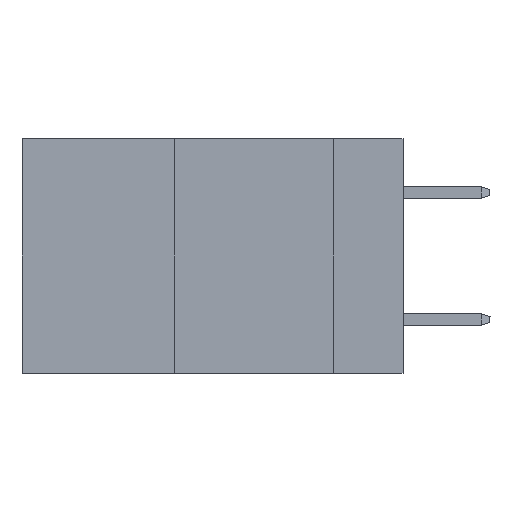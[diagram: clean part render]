
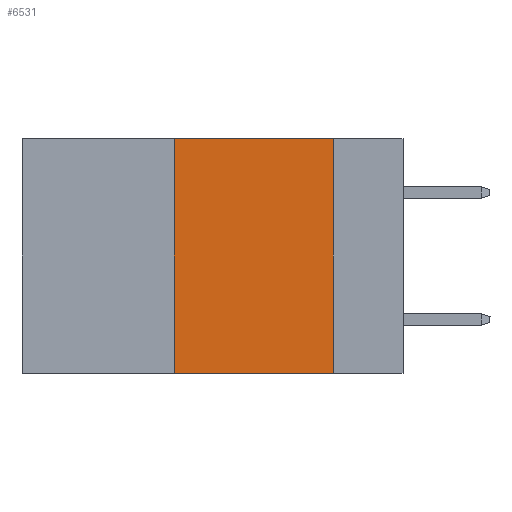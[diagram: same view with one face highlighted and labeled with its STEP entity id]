
A CAD part, left-side view. The second image highlights one B-rep face of the part: STEP entity #6531.
In plain terms, the highlighted planar face has unit normal (-1, 0, 0).
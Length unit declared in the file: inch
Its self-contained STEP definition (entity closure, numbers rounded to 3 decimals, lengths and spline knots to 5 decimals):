
#25 = EDGE_CURVE ( 'NONE', #2108, #4035, #2199, .T. ) ;
#592 = CARTESIAN_POINT ( 'NONE',  ( 0., 0.6, 0. ) ) ;
#597 = ORIENTED_EDGE ( 'NONE', *, *, #1719, .F. ) ;
#663 = DIRECTION ( 'NONE',  ( 0., 0., -1. ) ) ;
#950 = CARTESIAN_POINT ( 'NONE',  ( 0., 0.11, 0. ) ) ;
#1719 = EDGE_CURVE ( 'NONE', #12612, #11104, #5936, .T. ) ;
#2108 = VERTEX_POINT ( 'NONE', #12326 ) ;
#2199 = LINE ( 'NONE', #3392, #6156 ) ;
#3392 = CARTESIAN_POINT ( 'NONE',  ( 0., 0.6, -0.37 ) ) ;
#3549 = DIRECTION ( 'NONE',  ( 0., -1., 0. ) ) ;
#4035 = VERTEX_POINT ( 'NONE', #7643 ) ;
#4086 = FACE_OUTER_BOUND ( 'NONE', #12138, .T. ) ;
#4214 = EDGE_CURVE ( 'NONE', #2108, #12612, #14000, .T. ) ;
#4498 = CARTESIAN_POINT ( 'NONE',  ( 0., 0.36, 0. ) ) ;
#5598 = DIRECTION ( 'NONE',  ( 0., 0., -1. ) ) ;
#5936 = LINE ( 'NONE', #13459, #10824 ) ;
#6156 = VECTOR ( 'NONE', #8958, 39.37008 ) ;
#6178 = PLANE ( 'NONE',  #7375 ) ;
#6306 = DIRECTION ( 'NONE',  ( 0., 0., 1. ) ) ;
#6524 = VECTOR ( 'NONE', #5598, 39.37008 ) ;
#6531 = ADVANCED_FACE ( 'NONE', ( #4086 ), #6178, .F. ) ;
#6538 = LINE ( 'NONE', #950, #6524 ) ;
#6959 = VECTOR ( 'NONE', #6306, 39.37008 ) ;
#7375 = AXIS2_PLACEMENT_3D ( 'NONE', #592, #10593, #663 ) ;
#7643 = CARTESIAN_POINT ( 'NONE',  ( 0., 0.11, -0.37 ) ) ;
#7935 = ORIENTED_EDGE ( 'NONE', *, *, #4214, .F. ) ;
#8958 = DIRECTION ( 'NONE',  ( 0., -1., 0. ) ) ;
#10506 = CARTESIAN_POINT ( 'NONE',  ( 0., 0.11, 0. ) ) ;
#10593 = DIRECTION ( 'NONE',  ( 1., 0., 0. ) ) ;
#10824 = VECTOR ( 'NONE', #3549, 39.37008 ) ;
#11104 = VERTEX_POINT ( 'NONE', #10506 ) ;
#11786 = CARTESIAN_POINT ( 'NONE',  ( 0., 0.36, 0. ) ) ;
#11820 = ORIENTED_EDGE ( 'NONE', *, *, #25, .T. ) ;
#12138 = EDGE_LOOP ( 'NONE', ( #13128, #597, #7935, #11820 ) ) ;
#12326 = CARTESIAN_POINT ( 'NONE',  ( 0., 0.36, -0.37 ) ) ;
#12385 = EDGE_CURVE ( 'NONE', #11104, #4035, #6538, .T. ) ;
#12612 = VERTEX_POINT ( 'NONE', #4498 ) ;
#13128 = ORIENTED_EDGE ( 'NONE', *, *, #12385, .F. ) ;
#13459 = CARTESIAN_POINT ( 'NONE',  ( 0., 0.6, 0. ) ) ;
#14000 = LINE ( 'NONE', #11786, #6959 ) ;
